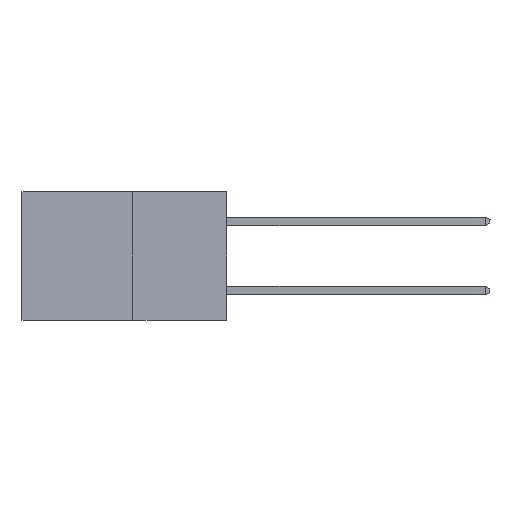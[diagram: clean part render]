
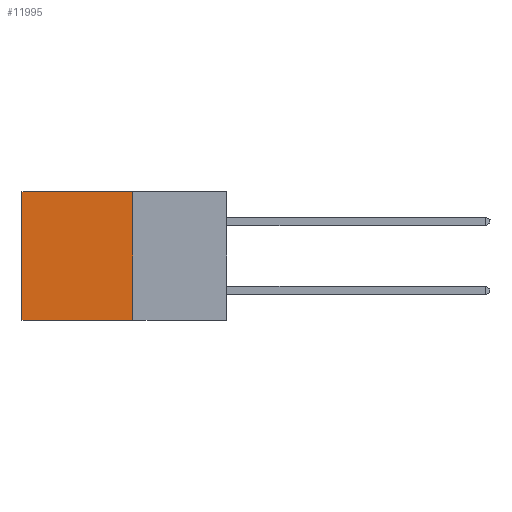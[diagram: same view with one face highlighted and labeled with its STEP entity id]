
A CAD part, left-side view. The second image highlights one B-rep face of the part: STEP entity #11995.
In plain terms, the highlighted planar face has unit normal (-1, 0, 0).
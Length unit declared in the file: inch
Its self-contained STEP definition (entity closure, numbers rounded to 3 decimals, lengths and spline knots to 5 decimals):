
#38 = ORIENTED_EDGE ( 'NONE', *, *, #12270, .T. ) ;
#233 = LINE ( 'NONE', #3943, #6243 ) ;
#424 = VERTEX_POINT ( 'NONE', #12853 ) ;
#817 = FACE_OUTER_BOUND ( 'NONE', #5575, .T. ) ;
#1041 = EDGE_CURVE ( 'NONE', #6986, #11129, #2336, .T. ) ;
#1939 = VECTOR ( 'NONE', #5253, 39.37008 ) ;
#2172 = AXIS2_PLACEMENT_3D ( 'NONE', #2222, #10417, #3480 ) ;
#2222 = CARTESIAN_POINT ( 'NONE',  ( 0.277, 0.27, -0.37 ) ) ;
#2336 = LINE ( 'NONE', #4893, #1939 ) ;
#2484 = VERTEX_POINT ( 'NONE', #8717 ) ;
#2985 = EDGE_CURVE ( 'NONE', #2484, #11129, #8544, .T. ) ;
#3084 = LINE ( 'NONE', #5727, #5833 ) ;
#3480 = DIRECTION ( 'NONE',  ( 0., 0., -1. ) ) ;
#3943 = CARTESIAN_POINT ( 'NONE',  ( 0.277, 0.27, 0. ) ) ;
#4182 = CARTESIAN_POINT ( 'NONE',  ( 0.277, 0.27, -0.37 ) ) ;
#4202 = DIRECTION ( 'NONE',  ( 0., 1., 0. ) ) ;
#4519 = ORIENTED_EDGE ( 'NONE', *, *, #2985, .F. ) ;
#4790 = CARTESIAN_POINT ( 'NONE',  ( 0.277, 0.59, 0. ) ) ;
#4893 = CARTESIAN_POINT ( 'NONE',  ( 0.277, 0.59, -0.37 ) ) ;
#5253 = DIRECTION ( 'NONE',  ( 0., 0., -1. ) ) ;
#5575 = EDGE_LOOP ( 'NONE', ( #6580, #4519, #9067, #38 ) ) ;
#5727 = CARTESIAN_POINT ( 'NONE',  ( 0.277, 0.27, -0.37 ) ) ;
#5833 = VECTOR ( 'NONE', #10368, 39.37008 ) ;
#6243 = VECTOR ( 'NONE', #10873, 39.37008 ) ;
#6580 = ORIENTED_EDGE ( 'NONE', *, *, #1041, .T. ) ;
#6617 = CARTESIAN_POINT ( 'NONE',  ( 0.277, 0.59, -0.37 ) ) ;
#6986 = VERTEX_POINT ( 'NONE', #4790 ) ;
#8170 = VECTOR ( 'NONE', #4202, 39.37008 ) ;
#8544 = LINE ( 'NONE', #4182, #8170 ) ;
#8717 = CARTESIAN_POINT ( 'NONE',  ( 0.277, 0.27, -0.37 ) ) ;
#9067 = ORIENTED_EDGE ( 'NONE', *, *, #13593, .F. ) ;
#10368 = DIRECTION ( 'NONE',  ( 0., 0., -1. ) ) ;
#10417 = DIRECTION ( 'NONE',  ( 1., 0., 0. ) ) ;
#10873 = DIRECTION ( 'NONE',  ( 0., 1., 0. ) ) ;
#11129 = VERTEX_POINT ( 'NONE', #6617 ) ;
#11995 = ADVANCED_FACE ( 'NONE', ( #817 ), #13802, .F. ) ;
#12270 = EDGE_CURVE ( 'NONE', #424, #6986, #233, .T. ) ;
#12853 = CARTESIAN_POINT ( 'NONE',  ( 0.277, 0.27, 0. ) ) ;
#13593 = EDGE_CURVE ( 'NONE', #424, #2484, #3084, .T. ) ;
#13802 = PLANE ( 'NONE',  #2172 ) ;
